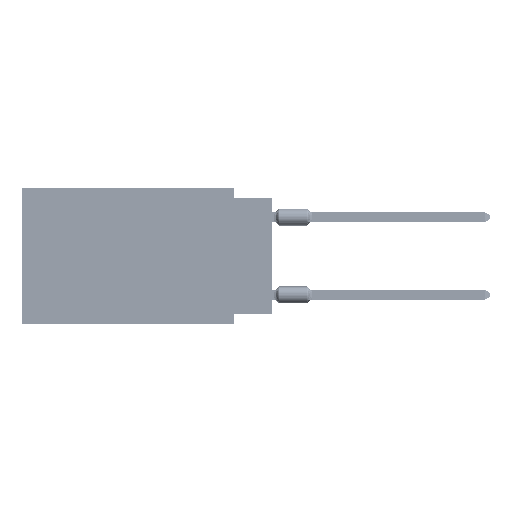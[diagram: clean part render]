
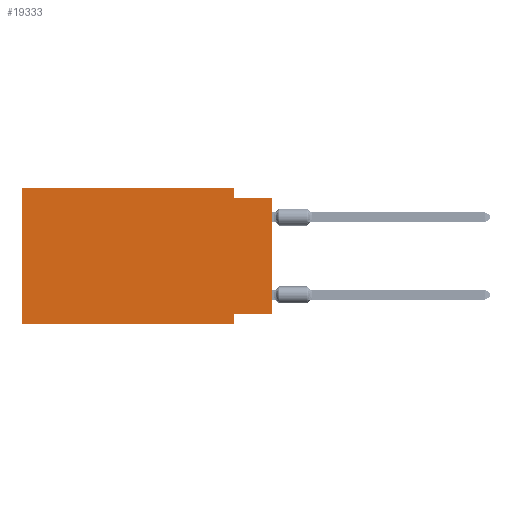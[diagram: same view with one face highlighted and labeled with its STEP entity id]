
A CAD part, left-side view. The second image highlights one B-rep face of the part: STEP entity #19333.
In plain terms, the highlighted planar face has unit normal (-1, 0, 0).
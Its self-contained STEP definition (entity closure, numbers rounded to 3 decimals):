
#163 = DIRECTION ( 'NONE',  ( 0., 0., -1. ) ) ;
#495 = LINE ( 'NONE', #76989, #16911 ) ;
#1440 = DIRECTION ( 'NONE',  ( 0., 0., -1. ) ) ;
#1929 = LINE ( 'NONE', #87500, #14476 ) ;
#2862 = EDGE_CURVE ( 'NONE', #89076, #97177, #61453, .T. ) ;
#7227 = EDGE_CURVE ( 'NONE', #97963, #80648, #1929, .T. ) ;
#7610 = DIRECTION ( 'NONE',  ( 0., -1., 0. ) ) ;
#8638 = ORIENTED_EDGE ( 'NONE', *, *, #7227, .F. ) ;
#10480 = LINE ( 'NONE', #48991, #67450 ) ;
#11417 = CARTESIAN_POINT ( 'NONE',  ( 0., 16.383, -8.89 ) ) ;
#13712 = CARTESIAN_POINT ( 'NONE',  ( 0., 0., -0.635 ) ) ;
#14476 = VECTOR ( 'NONE', #1440, 1000. ) ;
#15123 = EDGE_CURVE ( 'NONE', #67576, #97963, #57954, .T. ) ;
#16911 = VECTOR ( 'NONE', #7610, 1000. ) ;
#18871 = EDGE_CURVE ( 'NONE', #80648, #99122, #38520, .T. ) ;
#19333 = ADVANCED_FACE ( 'NONE', ( #30806 ), #44006, .F. ) ;
#19957 = CARTESIAN_POINT ( 'NONE',  ( 0., 16.383, 0. ) ) ;
#20379 = EDGE_CURVE ( 'NONE', #62691, #99122, #66025, .T. ) ;
#24356 = EDGE_CURVE ( 'NONE', #38673, #67576, #77794, .T. ) ;
#26580 = VECTOR ( 'NONE', #163, 1000. ) ;
#30806 = FACE_OUTER_BOUND ( 'NONE', #98017, .T. ) ;
#33708 = VECTOR ( 'NONE', #81223, 1000. ) ;
#36639 = DIRECTION ( 'NONE',  ( 0., 0., 1. ) ) ;
#37410 = CARTESIAN_POINT ( 'NONE',  ( 0., 16.383, 0. ) ) ;
#38520 = LINE ( 'NONE', #13712, #71387 ) ;
#38673 = VERTEX_POINT ( 'NONE', #11417 ) ;
#41907 = CARTESIAN_POINT ( 'NONE',  ( 0., 2.54, 0. ) ) ;
#44006 = PLANE ( 'NONE',  #69822 ) ;
#44588 = CARTESIAN_POINT ( 'NONE',  ( 0., 0., -8.255 ) ) ;
#45947 = CARTESIAN_POINT ( 'NONE',  ( 0., 16.383, 0. ) ) ;
#48549 = VECTOR ( 'NONE', #93965, 1000. ) ;
#48991 = CARTESIAN_POINT ( 'NONE',  ( 0., 0., -8.255 ) ) ;
#50340 = CARTESIAN_POINT ( 'NONE',  ( 0., 0., 0. ) ) ;
#57954 = LINE ( 'NONE', #19957, #33708 ) ;
#59958 = CARTESIAN_POINT ( 'NONE',  ( 0., 2.54, -8.89 ) ) ;
#61453 = LINE ( 'NONE', #59958, #26580 ) ;
#62597 = CARTESIAN_POINT ( 'NONE',  ( 0., 16.383, 0. ) ) ;
#62691 = VERTEX_POINT ( 'NONE', #44588 ) ;
#65926 = CARTESIAN_POINT ( 'NONE',  ( 0., 2.54, -8.89 ) ) ;
#66025 = LINE ( 'NONE', #50340, #78035 ) ;
#67450 = VECTOR ( 'NONE', #96570, 1000. ) ;
#67576 = VERTEX_POINT ( 'NONE', #45947 ) ;
#67791 = DIRECTION ( 'NONE',  ( 0., 0., -1. ) ) ;
#69822 = AXIS2_PLACEMENT_3D ( 'NONE', #37410, #88815, #67791 ) ;
#71387 = VECTOR ( 'NONE', #75490, 1000. ) ;
#75490 = DIRECTION ( 'NONE',  ( 0., -1., 0. ) ) ;
#76989 = CARTESIAN_POINT ( 'NONE',  ( 0., 16.383, -8.89 ) ) ;
#77794 = LINE ( 'NONE', #62597, #48549 ) ;
#78035 = VECTOR ( 'NONE', #36639, 1000. ) ;
#78128 = ORIENTED_EDGE ( 'NONE', *, *, #20379, .T. ) ;
#78938 = ORIENTED_EDGE ( 'NONE', *, *, #18871, .F. ) ;
#80648 = VERTEX_POINT ( 'NONE', #86312 ) ;
#81223 = DIRECTION ( 'NONE',  ( 0., -1., 0. ) ) ;
#86199 = ORIENTED_EDGE ( 'NONE', *, *, #15123, .F. ) ;
#86312 = CARTESIAN_POINT ( 'NONE',  ( 0., 2.54, -0.635 ) ) ;
#86893 = ORIENTED_EDGE ( 'NONE', *, *, #97899, .F. ) ;
#87084 = ORIENTED_EDGE ( 'NONE', *, *, #2862, .F. ) ;
#87370 = CARTESIAN_POINT ( 'NONE',  ( 0., 0., -0.635 ) ) ;
#87500 = CARTESIAN_POINT ( 'NONE',  ( 0., 2.54, 0. ) ) ;
#88815 = DIRECTION ( 'NONE',  ( 1., 0., 0. ) ) ;
#88836 = ORIENTED_EDGE ( 'NONE', *, *, #24356, .F. ) ;
#89076 = VERTEX_POINT ( 'NONE', #97042 ) ;
#93311 = EDGE_CURVE ( 'NONE', #38673, #97177, #495, .T. ) ;
#93965 = DIRECTION ( 'NONE',  ( 0., 0., 1. ) ) ;
#95062 = ORIENTED_EDGE ( 'NONE', *, *, #93311, .T. ) ;
#96570 = DIRECTION ( 'NONE',  ( 0., 1., 0. ) ) ;
#97042 = CARTESIAN_POINT ( 'NONE',  ( 0., 2.54, -8.255 ) ) ;
#97177 = VERTEX_POINT ( 'NONE', #65926 ) ;
#97899 = EDGE_CURVE ( 'NONE', #62691, #89076, #10480, .T. ) ;
#97963 = VERTEX_POINT ( 'NONE', #41907 ) ;
#98017 = EDGE_LOOP ( 'NONE', ( #78128, #78938, #8638, #86199, #88836, #95062, #87084, #86893 ) ) ;
#99122 = VERTEX_POINT ( 'NONE', #87370 ) ;
